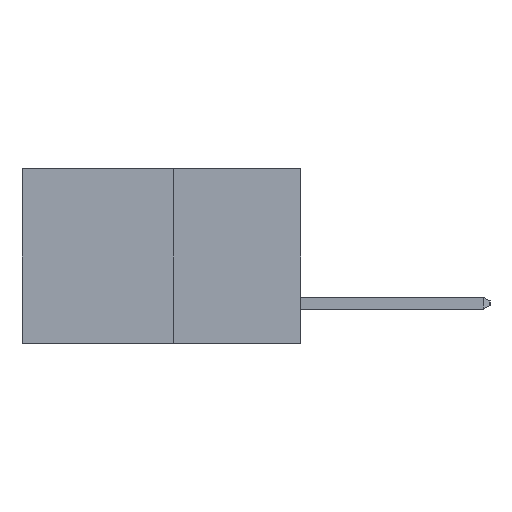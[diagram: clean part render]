
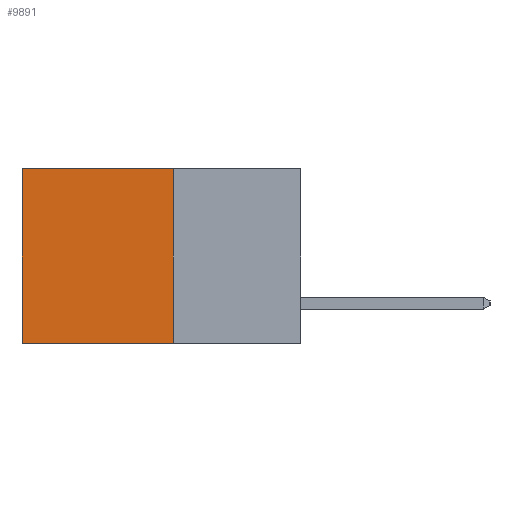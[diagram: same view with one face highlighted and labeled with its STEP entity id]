
A CAD part, left-side view. The second image highlights one B-rep face of the part: STEP entity #9891.
In plain terms, the highlighted planar face has unit normal (-1, 0, 0).
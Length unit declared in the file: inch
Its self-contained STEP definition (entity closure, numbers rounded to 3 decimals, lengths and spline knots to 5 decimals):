
#265 = LINE ( 'NONE', #7054, #6441 ) ;
#757 = CARTESIAN_POINT ( 'NONE',  ( 0.277, 0.27, -0.37 ) ) ;
#808 = CARTESIAN_POINT ( 'NONE',  ( 0.277, 0.27, 0. ) ) ;
#1445 = FACE_OUTER_BOUND ( 'NONE', #5474, .T. ) ;
#1468 = VECTOR ( 'NONE', #6509, 39.37008 ) ;
#1571 = DIRECTION ( 'NONE',  ( 0., 1., 0. ) ) ;
#2007 = EDGE_CURVE ( 'NONE', #3899, #3214, #8657, .T. ) ;
#2407 = DIRECTION ( 'NONE',  ( 0., 0., -1. ) ) ;
#2529 = VECTOR ( 'NONE', #5238, 39.37008 ) ;
#2562 = CARTESIAN_POINT ( 'NONE',  ( 0.277, 0.27, 0. ) ) ;
#2628 = CARTESIAN_POINT ( 'NONE',  ( 0.277, 0.27, -0.37 ) ) ;
#2791 = LINE ( 'NONE', #808, #8671 ) ;
#3084 = CARTESIAN_POINT ( 'NONE',  ( 0.277, 0.27, -0.37 ) ) ;
#3214 = VERTEX_POINT ( 'NONE', #8268 ) ;
#3874 = DIRECTION ( 'NONE',  ( 0., 0., -1. ) ) ;
#3899 = VERTEX_POINT ( 'NONE', #757 ) ;
#3992 = ORIENTED_EDGE ( 'NONE', *, *, #7689, .T. ) ;
#4259 = ORIENTED_EDGE ( 'NONE', *, *, #2007, .F. ) ;
#4449 = VERTEX_POINT ( 'NONE', #9110 ) ;
#4489 = CARTESIAN_POINT ( 'NONE',  ( 0.277, 0.27, -0.37 ) ) ;
#5238 = DIRECTION ( 'NONE',  ( 0., 1., 0. ) ) ;
#5474 = EDGE_LOOP ( 'NONE', ( #6528, #4259, #7650, #3992 ) ) ;
#6441 = VECTOR ( 'NONE', #2407, 39.37008 ) ;
#6509 = DIRECTION ( 'NONE',  ( 0., 0., -1. ) ) ;
#6528 = ORIENTED_EDGE ( 'NONE', *, *, #7743, .T. ) ;
#7054 = CARTESIAN_POINT ( 'NONE',  ( 0.277, 0.59, -0.37 ) ) ;
#7206 = VERTEX_POINT ( 'NONE', #2562 ) ;
#7650 = ORIENTED_EDGE ( 'NONE', *, *, #8970, .F. ) ;
#7689 = EDGE_CURVE ( 'NONE', #7206, #4449, #2791, .T. ) ;
#7712 = PLANE ( 'NONE',  #9317 ) ;
#7743 = EDGE_CURVE ( 'NONE', #4449, #3214, #265, .T. ) ;
#8268 = CARTESIAN_POINT ( 'NONE',  ( 0.277, 0.59, -0.37 ) ) ;
#8469 = DIRECTION ( 'NONE',  ( 1., 0., 0. ) ) ;
#8657 = LINE ( 'NONE', #4489, #2529 ) ;
#8671 = VECTOR ( 'NONE', #1571, 39.37008 ) ;
#8970 = EDGE_CURVE ( 'NONE', #7206, #3899, #9623, .T. ) ;
#9110 = CARTESIAN_POINT ( 'NONE',  ( 0.277, 0.59, 0. ) ) ;
#9317 = AXIS2_PLACEMENT_3D ( 'NONE', #3084, #8469, #3874 ) ;
#9623 = LINE ( 'NONE', #2628, #1468 ) ;
#9891 = ADVANCED_FACE ( 'NONE', ( #1445 ), #7712, .F. ) ;
